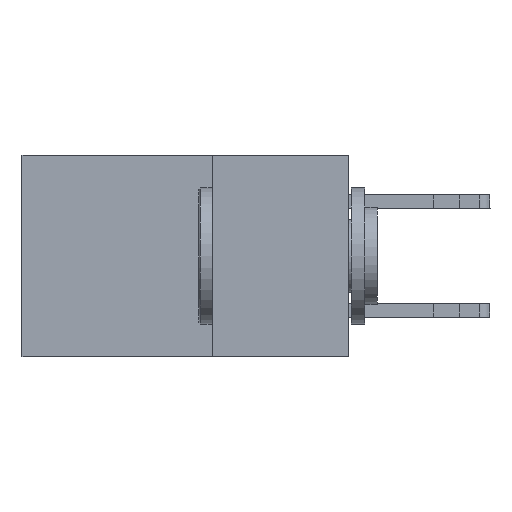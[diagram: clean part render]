
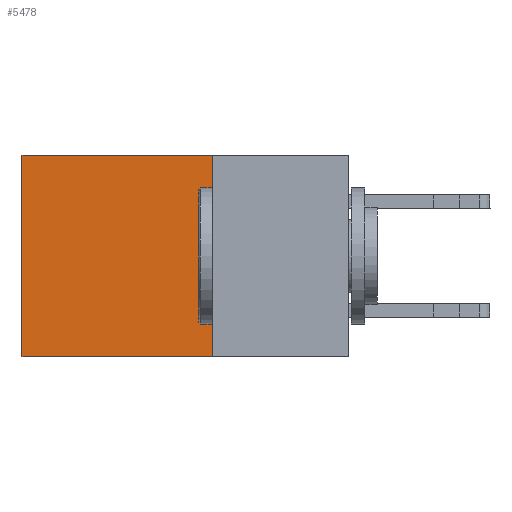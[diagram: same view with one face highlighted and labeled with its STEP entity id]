
A CAD part, left-side view. The second image highlights one B-rep face of the part: STEP entity #5478.
In plain terms, the highlighted planar face has unit normal (-1, 0, 0).
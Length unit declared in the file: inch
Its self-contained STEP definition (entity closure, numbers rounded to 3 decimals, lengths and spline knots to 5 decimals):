
#108 = EDGE_CURVE ( 'NONE', #2264, #1388, #6202, .T. ) ;
#505 = CARTESIAN_POINT ( 'NONE',  ( 0.2615, 0.25, -0.37 ) ) ;
#873 = EDGE_CURVE ( 'NONE', #1505, #5596, #5735, .T. ) ;
#1181 = LINE ( 'NONE', #4608, #12794 ) ;
#1388 = VERTEX_POINT ( 'NONE', #505 ) ;
#1505 = VERTEX_POINT ( 'NONE', #6647 ) ;
#2080 = VECTOR ( 'NONE', #6865, 39.37008 ) ;
#2264 = VERTEX_POINT ( 'NONE', #4228 ) ;
#3268 = DIRECTION ( 'NONE',  ( 0., 0., -1. ) ) ;
#3505 = CARTESIAN_POINT ( 'NONE',  ( 0.2615, 0.6, -0.37 ) ) ;
#3571 = ORIENTED_EDGE ( 'NONE', *, *, #873, .T. ) ;
#3603 = LINE ( 'NONE', #4801, #11299 ) ;
#3610 = EDGE_LOOP ( 'NONE', ( #3571, #10520, #9860, #11011 ) ) ;
#4228 = CARTESIAN_POINT ( 'NONE',  ( 0.2615, 0.25, 0. ) ) ;
#4608 = CARTESIAN_POINT ( 'NONE',  ( 0.2615, 0.25, -0.37 ) ) ;
#4801 = CARTESIAN_POINT ( 'NONE',  ( 0.2615, 0.25, 0. ) ) ;
#4893 = VECTOR ( 'NONE', #8487, 39.37008 ) ;
#5478 = ADVANCED_FACE ( 'NONE', ( #7680 ), #12787, .F. ) ;
#5596 = VERTEX_POINT ( 'NONE', #11037 ) ;
#5735 = LINE ( 'NONE', #3505, #2080 ) ;
#5767 = DIRECTION ( 'NONE',  ( 0., 1., 0. ) ) ;
#5899 = EDGE_CURVE ( 'NONE', #2264, #1505, #3603, .T. ) ;
#6202 = LINE ( 'NONE', #10528, #4893 ) ;
#6630 = DIRECTION ( 'NONE',  ( 1., 0., 0. ) ) ;
#6647 = CARTESIAN_POINT ( 'NONE',  ( 0.2615, 0.6, 0. ) ) ;
#6865 = DIRECTION ( 'NONE',  ( 0., 0., -1. ) ) ;
#7474 = CARTESIAN_POINT ( 'NONE',  ( 0.2615, 0.25, -0.37 ) ) ;
#7680 = FACE_OUTER_BOUND ( 'NONE', #3610, .T. ) ;
#8487 = DIRECTION ( 'NONE',  ( 0., 0., -1. ) ) ;
#9064 = EDGE_CURVE ( 'NONE', #1388, #5596, #1181, .T. ) ;
#9708 = DIRECTION ( 'NONE',  ( 0., 1., 0. ) ) ;
#9860 = ORIENTED_EDGE ( 'NONE', *, *, #108, .F. ) ;
#10520 = ORIENTED_EDGE ( 'NONE', *, *, #9064, .F. ) ;
#10528 = CARTESIAN_POINT ( 'NONE',  ( 0.2615, 0.25, -0.37 ) ) ;
#11011 = ORIENTED_EDGE ( 'NONE', *, *, #5899, .T. ) ;
#11037 = CARTESIAN_POINT ( 'NONE',  ( 0.2615, 0.6, -0.37 ) ) ;
#11299 = VECTOR ( 'NONE', #5767, 39.37008 ) ;
#12787 = PLANE ( 'NONE',  #13491 ) ;
#12794 = VECTOR ( 'NONE', #9708, 39.37008 ) ;
#13491 = AXIS2_PLACEMENT_3D ( 'NONE', #7474, #6630, #3268 ) ;
